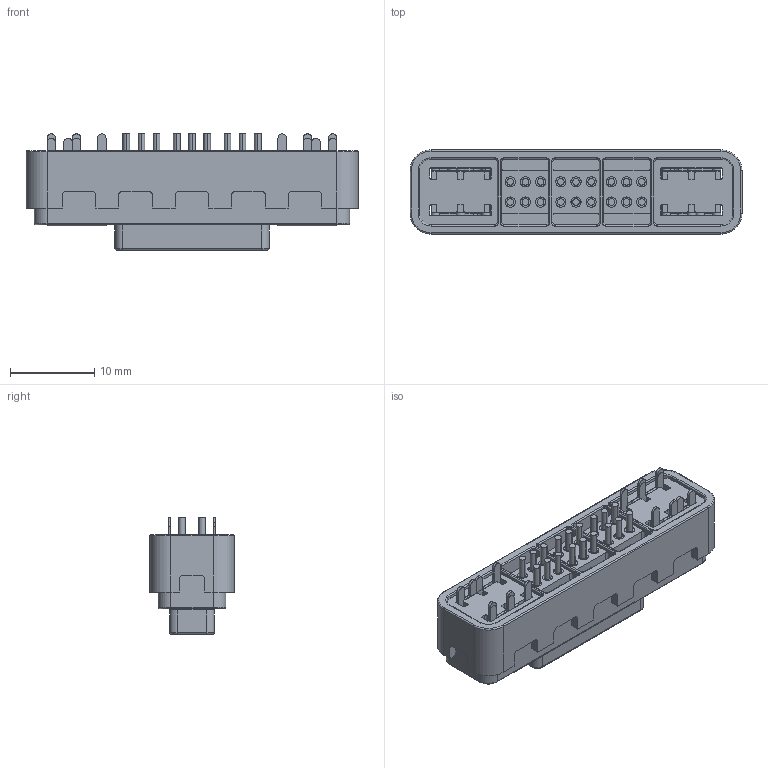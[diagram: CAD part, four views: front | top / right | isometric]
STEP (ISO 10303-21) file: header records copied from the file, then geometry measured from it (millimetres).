
FILE_DESCRIPTION (( 'STEP AP203' ), '1' );
FILE_NAME ('686A1821F20111E.STEP', '2023-04-21T14:57:41', ( 'Magnum' ), ( '' ), 'SwSTEP 2.0', 'SolidWorks 2020', '' );
FILE_SCHEMA (( 'CONFIG_CONTROL_DESIGN' ));
Length unit declared in the file: millimetre
Products named in the file (1): 686A1821F20111E
Bounding box: 39.4 x 10 x 13.8 mm (x, y, z)
Surface area: 8439.3 mm2
Topology: 20 solids, 20 shells, 1178 faces, 3076 edges, 1910 vertices
Faces by surface type: cylinder 552, plane 478, torus 80, sphere 68
Entity records: 35819 total; most frequent: DIRECTION 6618, CARTESIAN_POINT 6061, ORIENTED_EDGE 5980, EDGE_CURVE 2990, AXIS2_PLACEMENT_3D 2449, VERTEX_POINT 1892, LINE 1720, VECTOR 1720
